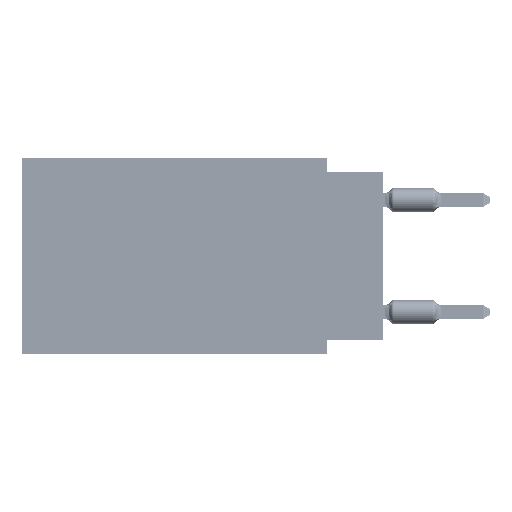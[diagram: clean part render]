
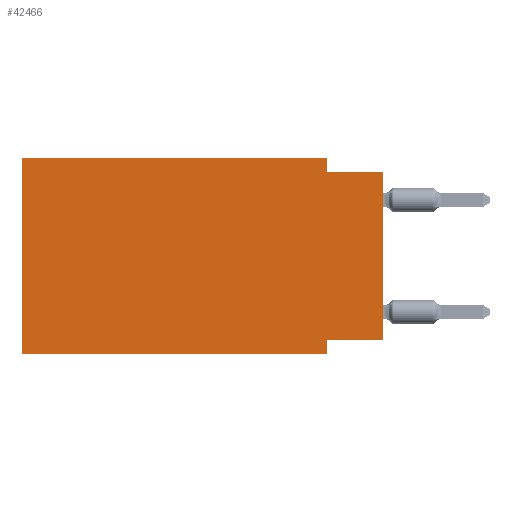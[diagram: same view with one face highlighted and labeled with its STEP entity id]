
A CAD part, left-side view. The second image highlights one B-rep face of the part: STEP entity #42466.
In plain terms, the highlighted planar face has unit normal (-1, 0, 0).
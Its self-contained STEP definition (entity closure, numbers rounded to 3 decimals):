
#1448 = LINE ( 'NONE', #38532, #61983 ) ;
#1461 = LINE ( 'NONE', #36890, #16723 ) ;
#1866 = VECTOR ( 'NONE', #18034, 1000. ) ;
#2680 = LINE ( 'NONE', #13042, #1866 ) ;
#3325 = DIRECTION ( 'NONE',  ( 1., 0., 0. ) ) ;
#6960 = VERTEX_POINT ( 'NONE', #63275 ) ;
#8199 = VERTEX_POINT ( 'NONE', #22458 ) ;
#8285 = LINE ( 'NONE', #65104, #60151 ) ;
#11009 = LINE ( 'NONE', #15362, #53084 ) ;
#11064 = EDGE_CURVE ( 'NONE', #14654, #8199, #2680, .T. ) ;
#12425 = DIRECTION ( 'NONE',  ( 0., 1., 0. ) ) ;
#13042 = CARTESIAN_POINT ( 'NONE',  ( 0., 0., -0.635 ) ) ;
#14654 = VERTEX_POINT ( 'NONE', #36596 ) ;
#14988 = PLANE ( 'NONE',  #18260 ) ;
#15362 = CARTESIAN_POINT ( 'NONE',  ( 0., 2.54, -8.89 ) ) ;
#16667 = CARTESIAN_POINT ( 'NONE',  ( 0., 16.383, 0. ) ) ;
#16723 = VECTOR ( 'NONE', #27180, 1000. ) ;
#18034 = DIRECTION ( 'NONE',  ( 0., -1., 0. ) ) ;
#18260 = AXIS2_PLACEMENT_3D ( 'NONE', #19666, #3325, #29689 ) ;
#19666 = CARTESIAN_POINT ( 'NONE',  ( 0., 16.383, 0. ) ) ;
#19953 = DIRECTION ( 'NONE',  ( 0., -1., 0. ) ) ;
#21562 = DIRECTION ( 'NONE',  ( 0., 0., -1. ) ) ;
#21942 = VECTOR ( 'NONE', #12425, 1000. ) ;
#22458 = CARTESIAN_POINT ( 'NONE',  ( 0., 0., -0.635 ) ) ;
#22785 = EDGE_CURVE ( 'NONE', #31387, #60288, #37847, .T. ) ;
#24282 = ORIENTED_EDGE ( 'NONE', *, *, #31800, .F. ) ;
#24857 = EDGE_CURVE ( 'NONE', #6960, #14654, #63331, .T. ) ;
#26563 = ORIENTED_EDGE ( 'NONE', *, *, #58889, .F. ) ;
#26860 = CARTESIAN_POINT ( 'NONE',  ( 0., 2.54, -8.89 ) ) ;
#27105 = VERTEX_POINT ( 'NONE', #35057 ) ;
#27180 = DIRECTION ( 'NONE',  ( 0., 0., 1. ) ) ;
#27895 = EDGE_CURVE ( 'NONE', #27105, #60438, #8285, .T. ) ;
#29689 = DIRECTION ( 'NONE',  ( 0., 0., -1. ) ) ;
#30283 = ORIENTED_EDGE ( 'NONE', *, *, #60194, .F. ) ;
#30557 = DIRECTION ( 'NONE',  ( 0., -1., 0. ) ) ;
#30974 = ORIENTED_EDGE ( 'NONE', *, *, #24857, .F. ) ;
#31037 = EDGE_LOOP ( 'NONE', ( #56398, #58835, #30974, #30283, #24282, #57705, #26563, #43511 ) ) ;
#31387 = VERTEX_POINT ( 'NONE', #46230 ) ;
#31389 = DIRECTION ( 'NONE',  ( 0., 0., -1. ) ) ;
#31800 = EDGE_CURVE ( 'NONE', #27105, #47678, #1461, .T. ) ;
#34913 = CARTESIAN_POINT ( 'NONE',  ( 0., 2.54, -8.255 ) ) ;
#35057 = CARTESIAN_POINT ( 'NONE',  ( 0., 16.383, -8.89 ) ) ;
#35670 = EDGE_CURVE ( 'NONE', #31387, #8199, #1448, .T. ) ;
#36596 = CARTESIAN_POINT ( 'NONE',  ( 0., 2.54, -0.635 ) ) ;
#36890 = CARTESIAN_POINT ( 'NONE',  ( 0., 16.383, 0. ) ) ;
#37446 = VECTOR ( 'NONE', #21562, 1000. ) ;
#37847 = LINE ( 'NONE', #58231, #21942 ) ;
#37869 = DIRECTION ( 'NONE',  ( 0., 0., 1. ) ) ;
#38532 = CARTESIAN_POINT ( 'NONE',  ( 0., 0., 0. ) ) ;
#42466 = ADVANCED_FACE ( 'NONE', ( #60784 ), #14988, .F. ) ;
#42552 = VECTOR ( 'NONE', #30557, 1000. ) ;
#43511 = ORIENTED_EDGE ( 'NONE', *, *, #22785, .F. ) ;
#46230 = CARTESIAN_POINT ( 'NONE',  ( 0., 0., -8.255 ) ) ;
#47383 = CARTESIAN_POINT ( 'NONE',  ( 0., 16.383, 0. ) ) ;
#47678 = VERTEX_POINT ( 'NONE', #16667 ) ;
#51645 = CARTESIAN_POINT ( 'NONE',  ( 0., 2.54, 0. ) ) ;
#52415 = LINE ( 'NONE', #47383, #42552 ) ;
#53084 = VECTOR ( 'NONE', #31389, 1000. ) ;
#56398 = ORIENTED_EDGE ( 'NONE', *, *, #35670, .T. ) ;
#57705 = ORIENTED_EDGE ( 'NONE', *, *, #27895, .T. ) ;
#58231 = CARTESIAN_POINT ( 'NONE',  ( 0., 0., -8.255 ) ) ;
#58835 = ORIENTED_EDGE ( 'NONE', *, *, #11064, .F. ) ;
#58889 = EDGE_CURVE ( 'NONE', #60288, #60438, #11009, .T. ) ;
#60151 = VECTOR ( 'NONE', #19953, 1000. ) ;
#60194 = EDGE_CURVE ( 'NONE', #47678, #6960, #52415, .T. ) ;
#60288 = VERTEX_POINT ( 'NONE', #34913 ) ;
#60438 = VERTEX_POINT ( 'NONE', #26860 ) ;
#60784 = FACE_OUTER_BOUND ( 'NONE', #31037, .T. ) ;
#61983 = VECTOR ( 'NONE', #37869, 1000. ) ;
#63275 = CARTESIAN_POINT ( 'NONE',  ( 0., 2.54, 0. ) ) ;
#63331 = LINE ( 'NONE', #51645, #37446 ) ;
#65104 = CARTESIAN_POINT ( 'NONE',  ( 0., 16.383, -8.89 ) ) ;
